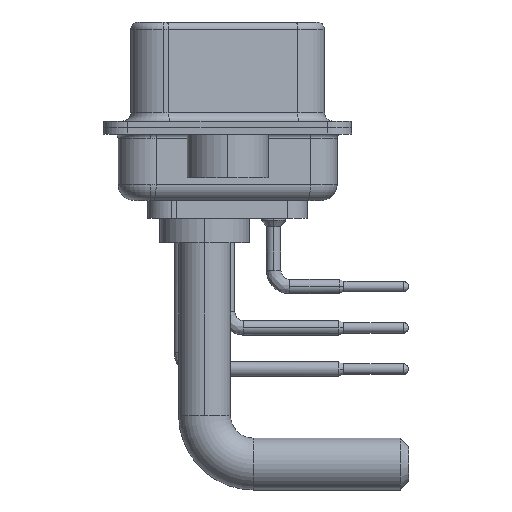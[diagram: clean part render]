
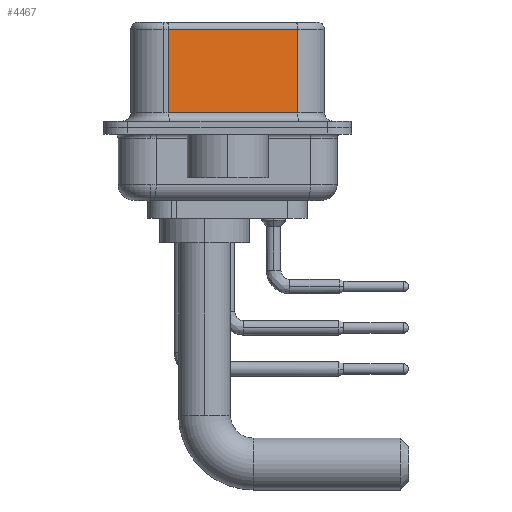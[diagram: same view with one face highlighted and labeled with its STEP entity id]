
A CAD part, left-side view. The second image highlights one B-rep face of the part: STEP entity #4467.
In plain terms, the highlighted planar face has unit normal (-0.985, -0.174, 0).
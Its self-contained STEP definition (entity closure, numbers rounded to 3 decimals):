
#940 = EDGE_CURVE ( 'NONE', #32175, #6132, #24008, .T. ) ;
#1353 = ORIENTED_EDGE ( 'NONE', *, *, #10221, .T. ) ;
#1924 = VECTOR ( 'NONE', #20457, 1000. ) ;
#2233 = VERTEX_POINT ( 'NONE', #16082 ) ;
#2303 = VECTOR ( 'NONE', #14580, 1000. ) ;
#2944 = EDGE_CURVE ( 'NONE', #14972, #32175, #32663, .T. ) ;
#3547 = VECTOR ( 'NONE', #29189, 1000. ) ;
#3682 = ORIENTED_EDGE ( 'NONE', *, *, #2944, .T. ) ;
#4294 = VECTOR ( 'NONE', #23941, 1000. ) ;
#4467 = ADVANCED_FACE ( 'NONE', ( #24166 ), #19622, .F. ) ;
#5129 = CARTESIAN_POINT ( 'NONE',  ( 5.132, -4.322, 0.9 ) ) ;
#6132 = VERTEX_POINT ( 'NONE', #29185 ) ;
#7138 = EDGE_LOOP ( 'NONE', ( #33736, #1353, #3682, #28424 ) ) ;
#7143 = CARTESIAN_POINT ( 'NONE',  ( 3.73, 3.628, 6.52 ) ) ;
#8383 = CARTESIAN_POINT ( 'NONE',  ( 3.73, 3.628, 0.9 ) ) ;
#9074 = CARTESIAN_POINT ( 'NONE',  ( 5.132, -4.322, 6.52 ) ) ;
#10221 = EDGE_CURVE ( 'NONE', #2233, #14972, #17515, .T. ) ;
#14580 = DIRECTION ( 'NONE',  ( -0.174, 0.985, 0. ) ) ;
#14972 = VERTEX_POINT ( 'NONE', #20304 ) ;
#16082 = CARTESIAN_POINT ( 'NONE',  ( 5.132, -4.322, 6.02 ) ) ;
#16853 = DIRECTION ( 'NONE',  ( 0.985, 0.174, 0. ) ) ;
#17515 = LINE ( 'NONE', #27751, #2303 ) ;
#19448 = DIRECTION ( 'NONE',  ( -0.174, 0.985, 0. ) ) ;
#19622 = PLANE ( 'NONE',  #23559 ) ;
#20304 = CARTESIAN_POINT ( 'NONE',  ( 3.73, 3.628, 6.02 ) ) ;
#20457 = DIRECTION ( 'NONE',  ( 0., 0., -1. ) ) ;
#23559 = AXIS2_PLACEMENT_3D ( 'NONE', #9074, #16853, #19448 ) ;
#23808 = EDGE_CURVE ( 'NONE', #2233, #6132, #31378, .T. ) ;
#23941 = DIRECTION ( 'NONE',  ( 0., 0., -1. ) ) ;
#24008 = LINE ( 'NONE', #5129, #3547 ) ;
#24166 = FACE_OUTER_BOUND ( 'NONE', #7138, .T. ) ;
#27751 = CARTESIAN_POINT ( 'NONE',  ( 5.132, -4.322, 6.02 ) ) ;
#28424 = ORIENTED_EDGE ( 'NONE', *, *, #940, .T. ) ;
#29185 = CARTESIAN_POINT ( 'NONE',  ( 5.132, -4.322, 0.9 ) ) ;
#29189 = DIRECTION ( 'NONE',  ( 0.174, -0.985, 0. ) ) ;
#29814 = CARTESIAN_POINT ( 'NONE',  ( 5.132, -4.322, 6.52 ) ) ;
#31378 = LINE ( 'NONE', #29814, #4294 ) ;
#32175 = VERTEX_POINT ( 'NONE', #8383 ) ;
#32663 = LINE ( 'NONE', #7143, #1924 ) ;
#33736 = ORIENTED_EDGE ( 'NONE', *, *, #23808, .F. ) ;
